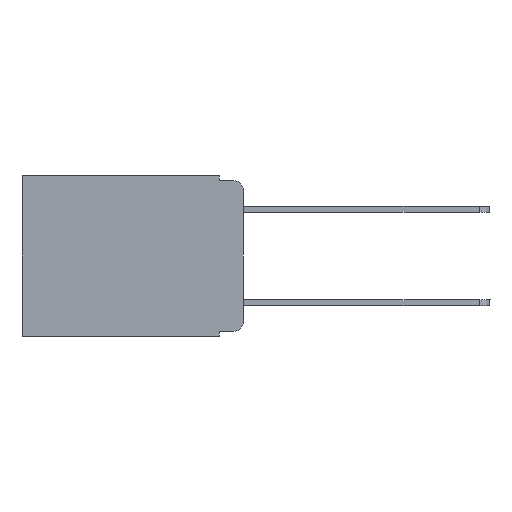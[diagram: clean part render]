
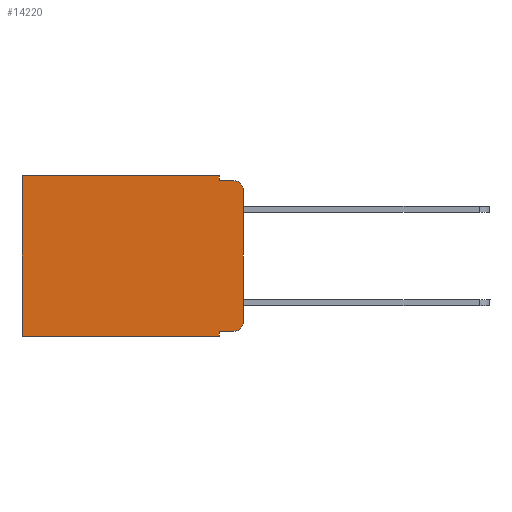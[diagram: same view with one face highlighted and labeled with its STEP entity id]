
A CAD part, left-side view. The second image highlights one B-rep face of the part: STEP entity #14220.
In plain terms, the highlighted planar face has unit normal (-1, 0, 0).
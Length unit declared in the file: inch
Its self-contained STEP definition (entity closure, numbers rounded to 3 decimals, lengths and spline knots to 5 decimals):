
#46 = DIRECTION ( 'NONE',  ( 0., -1., 0. ) ) ;
#78 = CARTESIAN_POINT ( 'NONE',  ( 0.298, 0.473, 0. ) ) ;
#139 = LINE ( 'NONE', #10961, #12865 ) ;
#145 = EDGE_CURVE ( 'NONE', #9391, #11457, #9073, .T. ) ;
#262 = CIRCLE ( 'NONE', #3295, 0.02 ) ;
#520 = CARTESIAN_POINT ( 'NONE',  ( 0.298, 0.473, 0. ) ) ;
#561 = ORIENTED_EDGE ( 'NONE', *, *, #8248, .T. ) ;
#669 = CARTESIAN_POINT ( 'NONE',  ( 0.298, 0., 0. ) ) ;
#820 = CARTESIAN_POINT ( 'NONE',  ( 0.298, 0.02, -0.333 ) ) ;
#913 = DIRECTION ( 'NONE',  ( 0., 0., -1. ) ) ;
#1408 = CARTESIAN_POINT ( 'NONE',  ( 0.298, 0.051, 0. ) ) ;
#1893 = CARTESIAN_POINT ( 'NONE',  ( 0.298, 0.051, 0. ) ) ;
#2025 = EDGE_CURVE ( 'NONE', #4178, #3699, #11407, .T. ) ;
#2051 = CARTESIAN_POINT ( 'NONE',  ( 0.298, 0.051, -0.01 ) ) ;
#2662 = VECTOR ( 'NONE', #13936, 39.37008 ) ;
#2664 = VERTEX_POINT ( 'NONE', #820 ) ;
#2949 = CARTESIAN_POINT ( 'NONE',  ( 0.298, 0.051, 0. ) ) ;
#3105 = DIRECTION ( 'NONE',  ( 0., 0., -1. ) ) ;
#3295 = AXIS2_PLACEMENT_3D ( 'NONE', #5490, #10453, #913 ) ;
#3444 = DIRECTION ( 'NONE',  ( 0., 1., 0. ) ) ;
#3498 = EDGE_CURVE ( 'NONE', #13260, #4182, #139, .T. ) ;
#3577 = ORIENTED_EDGE ( 'NONE', *, *, #10811, .F. ) ;
#3645 = VECTOR ( 'NONE', #3444, 39.37008 ) ;
#3695 = CARTESIAN_POINT ( 'NONE',  ( 0.298, 0.051, -0.333 ) ) ;
#3699 = VERTEX_POINT ( 'NONE', #11345 ) ;
#4043 = LINE ( 'NONE', #2949, #14935 ) ;
#4178 = VERTEX_POINT ( 'NONE', #78 ) ;
#4182 = VERTEX_POINT ( 'NONE', #9654 ) ;
#5104 = EDGE_LOOP ( 'NONE', ( #12326, #561, #9874, #3577, #12486, #7416, #8262, #10975, #15430, #14895 ) ) ;
#5263 = VERTEX_POINT ( 'NONE', #1408 ) ;
#5490 = CARTESIAN_POINT ( 'NONE',  ( 0.298, 0.02, -0.313 ) ) ;
#5587 = CARTESIAN_POINT ( 'NONE',  ( 0.298, 0., -0.313 ) ) ;
#6177 = AXIS2_PLACEMENT_3D ( 'NONE', #669, #10300, #3105 ) ;
#6326 = EDGE_CURVE ( 'NONE', #11457, #3699, #13001, .T. ) ;
#6408 = DIRECTION ( 'NONE',  ( 0., 0., -1. ) ) ;
#6669 = LINE ( 'NONE', #10298, #9572 ) ;
#7056 = CARTESIAN_POINT ( 'NONE',  ( 0.298, 0.051, -0.333 ) ) ;
#7416 = ORIENTED_EDGE ( 'NONE', *, *, #2025, .T. ) ;
#8013 = FACE_OUTER_BOUND ( 'NONE', #5104, .T. ) ;
#8047 = EDGE_CURVE ( 'NONE', #9005, #13737, #6669, .T. ) ;
#8248 = EDGE_CURVE ( 'NONE', #9005, #4182, #14786, .T. ) ;
#8262 = ORIENTED_EDGE ( 'NONE', *, *, #6326, .F. ) ;
#8526 = LINE ( 'NONE', #3695, #9096 ) ;
#8546 = EDGE_CURVE ( 'NONE', #9391, #2664, #8526, .T. ) ;
#8704 = DIRECTION ( 'NONE',  ( 0., -1., 0. ) ) ;
#8754 = CARTESIAN_POINT ( 'NONE',  ( 0.298, 0., 0. ) ) ;
#8888 = DIRECTION ( 'NONE',  ( 0., 0., -1. ) ) ;
#8911 = DIRECTION ( 'NONE',  ( 0., 0., -1. ) ) ;
#9005 = VERTEX_POINT ( 'NONE', #15583 ) ;
#9073 = LINE ( 'NONE', #1893, #2662 ) ;
#9096 = VECTOR ( 'NONE', #46, 39.37008 ) ;
#9134 = EDGE_CURVE ( 'NONE', #2664, #13737, #262, .T. ) ;
#9391 = VERTEX_POINT ( 'NONE', #7056 ) ;
#9572 = VECTOR ( 'NONE', #15092, 39.37008 ) ;
#9654 = CARTESIAN_POINT ( 'NONE',  ( 0.298, 0.02, -0.01 ) ) ;
#9874 = ORIENTED_EDGE ( 'NONE', *, *, #3498, .F. ) ;
#10298 = CARTESIAN_POINT ( 'NONE',  ( 0.298, 0., 0. ) ) ;
#10300 = DIRECTION ( 'NONE',  ( 1., 0., 0. ) ) ;
#10338 = DIRECTION ( 'NONE',  ( -1., 0., 0. ) ) ;
#10389 = VECTOR ( 'NONE', #8911, 39.37008 ) ;
#10453 = DIRECTION ( 'NONE',  ( -1., 0., 0. ) ) ;
#10811 = EDGE_CURVE ( 'NONE', #5263, #13260, #4043, .T. ) ;
#10961 = CARTESIAN_POINT ( 'NONE',  ( 0.298, 0.051, -0.01 ) ) ;
#10975 = ORIENTED_EDGE ( 'NONE', *, *, #145, .F. ) ;
#11160 = DIRECTION ( 'NONE',  ( 0., 1., 0. ) ) ;
#11250 = LINE ( 'NONE', #8754, #14245 ) ;
#11345 = CARTESIAN_POINT ( 'NONE',  ( 0.298, 0.473, -0.343 ) ) ;
#11407 = LINE ( 'NONE', #520, #10389 ) ;
#11457 = VERTEX_POINT ( 'NONE', #14921 ) ;
#12326 = ORIENTED_EDGE ( 'NONE', *, *, #8047, .F. ) ;
#12472 = CARTESIAN_POINT ( 'NONE',  ( 0.298, 0.02, -0.03 ) ) ;
#12486 = ORIENTED_EDGE ( 'NONE', *, *, #15344, .T. ) ;
#12865 = VECTOR ( 'NONE', #8704, 39.37008 ) ;
#13001 = LINE ( 'NONE', #14180, #3645 ) ;
#13260 = VERTEX_POINT ( 'NONE', #2051 ) ;
#13737 = VERTEX_POINT ( 'NONE', #5587 ) ;
#13936 = DIRECTION ( 'NONE',  ( 0., 0., -1. ) ) ;
#14043 = AXIS2_PLACEMENT_3D ( 'NONE', #12472, #10338, #6408 ) ;
#14146 = PLANE ( 'NONE',  #6177 ) ;
#14180 = CARTESIAN_POINT ( 'NONE',  ( 0.298, 0., -0.343 ) ) ;
#14220 = ADVANCED_FACE ( 'NONE', ( #8013 ), #14146, .F. ) ;
#14245 = VECTOR ( 'NONE', #11160, 39.37008 ) ;
#14786 = CIRCLE ( 'NONE', #14043, 0.02 ) ;
#14895 = ORIENTED_EDGE ( 'NONE', *, *, #9134, .T. ) ;
#14921 = CARTESIAN_POINT ( 'NONE',  ( 0.298, 0.051, -0.343 ) ) ;
#14935 = VECTOR ( 'NONE', #8888, 39.37008 ) ;
#15092 = DIRECTION ( 'NONE',  ( 0., 0., -1. ) ) ;
#15344 = EDGE_CURVE ( 'NONE', #5263, #4178, #11250, .T. ) ;
#15430 = ORIENTED_EDGE ( 'NONE', *, *, #8546, .T. ) ;
#15583 = CARTESIAN_POINT ( 'NONE',  ( 0.298, 0., -0.03 ) ) ;
